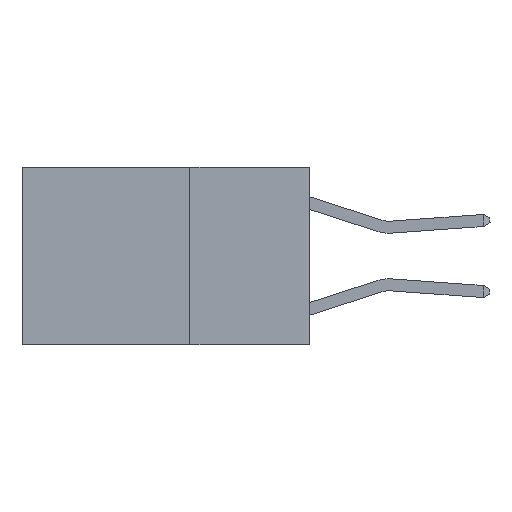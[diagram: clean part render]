
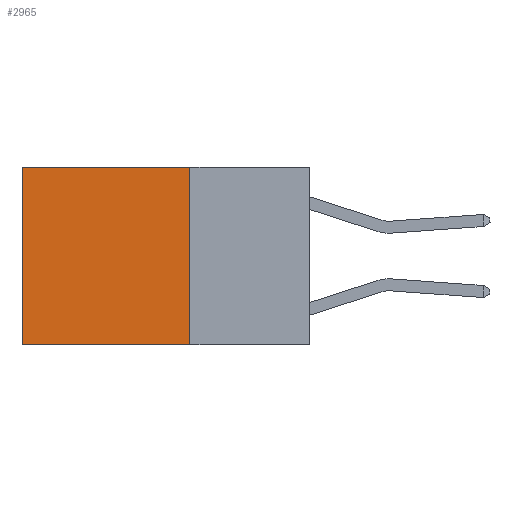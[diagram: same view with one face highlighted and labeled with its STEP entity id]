
A CAD part, left-side view. The second image highlights one B-rep face of the part: STEP entity #2965.
In plain terms, the highlighted planar face has unit normal (-1, 0, 0).
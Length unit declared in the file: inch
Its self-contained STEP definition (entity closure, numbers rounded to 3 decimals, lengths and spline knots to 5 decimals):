
#51 = ORIENTED_EDGE ( 'NONE', *, *, #5392, .T. ) ;
#114 = ORIENTED_EDGE ( 'NONE', *, *, #6216, .F. ) ;
#120 = ORIENTED_EDGE ( 'NONE', *, *, #3065, .F. ) ;
#191 = ORIENTED_EDGE ( 'NONE', *, *, #1427, .T. ) ;
#713 = EDGE_LOOP ( 'NONE', ( #51, #114, #120, #191 ) ) ;
#840 = CARTESIAN_POINT ( 'NONE',  ( 0.2625, 0.6, -0.37 ) ) ;
#1192 = VECTOR ( 'NONE', #1699, 39.37008 ) ;
#1427 = EDGE_CURVE ( 'NONE', #7644, #2552, #3559, .T. ) ;
#1699 = DIRECTION ( 'NONE',  ( 0., 0., -1. ) ) ;
#1820 = AXIS2_PLACEMENT_3D ( 'NONE', #6204, #1918, #6912 ) ;
#1918 = DIRECTION ( 'NONE',  ( 1., 0., 0. ) ) ;
#2281 = VECTOR ( 'NONE', #4179, 39.37008 ) ;
#2552 = VERTEX_POINT ( 'NONE', #6363 ) ;
#2761 = VECTOR ( 'NONE', #8659, 39.37008 ) ;
#2776 = CARTESIAN_POINT ( 'NONE',  ( 0.2625, 0.25, 0. ) ) ;
#2897 = LINE ( 'NONE', #3151, #1192 ) ;
#2965 = ADVANCED_FACE ( 'NONE', ( #5094 ), #4042, .F. ) ;
#3065 = EDGE_CURVE ( 'NONE', #7644, #3956, #4176, .T. ) ;
#3151 = CARTESIAN_POINT ( 'NONE',  ( 0.2625, 0.6, 0. ) ) ;
#3313 = VERTEX_POINT ( 'NONE', #840 ) ;
#3559 = LINE ( 'NONE', #5832, #5243 ) ;
#3623 = CARTESIAN_POINT ( 'NONE',  ( 0.2625, 0.25, 0. ) ) ;
#3895 = CARTESIAN_POINT ( 'NONE',  ( 0.2625, 0.25, -0.37 ) ) ;
#3956 = VERTEX_POINT ( 'NONE', #3895 ) ;
#4042 = PLANE ( 'NONE',  #1820 ) ;
#4176 = LINE ( 'NONE', #2776, #2281 ) ;
#4179 = DIRECTION ( 'NONE',  ( 0., 0., -1. ) ) ;
#4667 = LINE ( 'NONE', #7987, #2761 ) ;
#5094 = FACE_OUTER_BOUND ( 'NONE', #713, .T. ) ;
#5243 = VECTOR ( 'NONE', #6410, 39.37008 ) ;
#5392 = EDGE_CURVE ( 'NONE', #2552, #3313, #2897, .T. ) ;
#5832 = CARTESIAN_POINT ( 'NONE',  ( 0.2625, 0.25, 0. ) ) ;
#6204 = CARTESIAN_POINT ( 'NONE',  ( 0.2625, 0.25, 0. ) ) ;
#6216 = EDGE_CURVE ( 'NONE', #3956, #3313, #4667, .T. ) ;
#6363 = CARTESIAN_POINT ( 'NONE',  ( 0.2625, 0.6, 0. ) ) ;
#6410 = DIRECTION ( 'NONE',  ( 0., 1., 0. ) ) ;
#6912 = DIRECTION ( 'NONE',  ( 0., 0., -1. ) ) ;
#7644 = VERTEX_POINT ( 'NONE', #3623 ) ;
#7987 = CARTESIAN_POINT ( 'NONE',  ( 0.2625, 0.25, -0.37 ) ) ;
#8659 = DIRECTION ( 'NONE',  ( 0., 1., 0. ) ) ;
